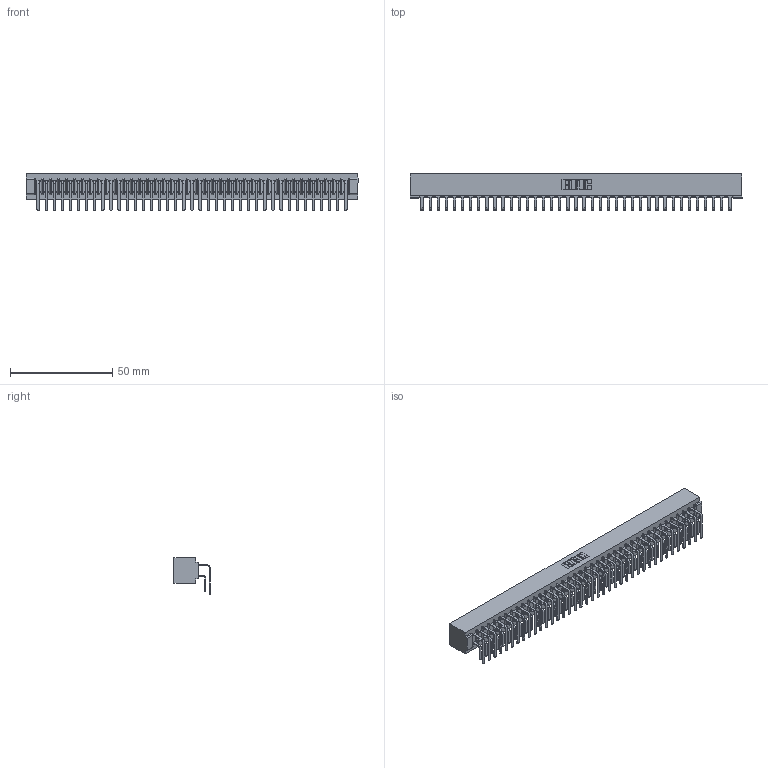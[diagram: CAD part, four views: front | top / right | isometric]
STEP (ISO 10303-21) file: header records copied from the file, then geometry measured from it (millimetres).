
FILE_DESCRIPTION (( 'STEP AP203' ), '1' );
FILE_NAME ('307-039-459-101.STEP', '2020-09-29T07:55:39', ( '' ), ( '' ), 'SwSTEP 2.0', 'SolidWorks 2020', '' );
FILE_SCHEMA (( 'CONFIG_CONTROL_DESIGN' ));
Length unit declared in the file: inch
Products named in the file (4): 307 Part_No Mounting Lugs; 307-290-001_559 - 2 (Single); 307-039-459-101; 307-290-001_558 559 - 1 (Single)
Assembly tree (79 placements, depth 2):
  307-039-459-101
    307 Part_No Mounting Lugs
    307-290-001_558 559 - 1 (Single)  x39
    307-290-001_559 - 2 (Single)  x39
Bounding box: 162.41 x 17.69 x 18.07 mm (x, y, z)
Volume: 18142.2 mm3; surface area: 24466.9 mm2
Topology: 79 solids, 79 shells, 4050 faces, 11375 edges, 7370 vertices
Faces by surface type: plane 2640, cylinder 1330, sphere 80
Entity records: 36221 total; most frequent: CARTESIAN_POINT 5925, ORIENTED_EDGE 5870, DIRECTION 5803, EDGE_CURVE 2935, VECTOR 2251, LINE 2251, VERTEX_POINT 1898, AXIS2_PLACEMENT_3D 1776
